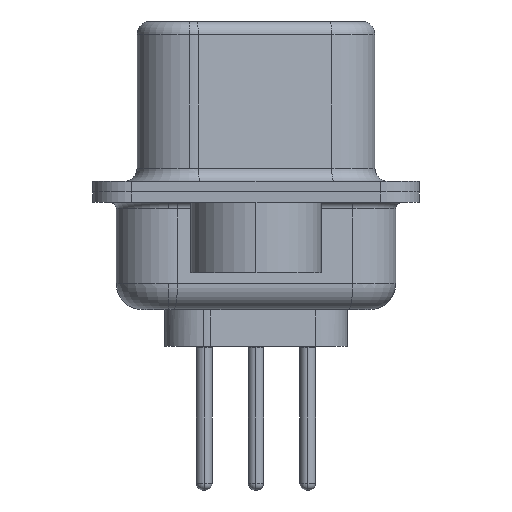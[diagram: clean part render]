
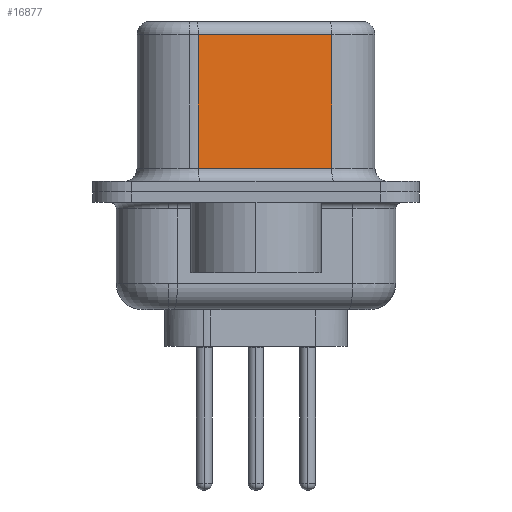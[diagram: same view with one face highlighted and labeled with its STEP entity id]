
A CAD part, left-side view. The second image highlights one B-rep face of the part: STEP entity #16877.
In plain terms, the highlighted planar face has unit normal (-0.985, -0.174, 0).
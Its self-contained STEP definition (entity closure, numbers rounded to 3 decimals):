
#751 = DIRECTION ( 'NONE',  ( 0.985, 0.174, 0. ) ) ;
#2518 = EDGE_CURVE ( 'NONE', #10097, #17260, #2590, .T. ) ;
#2590 = LINE ( 'NONE', #4401, #18952 ) ;
#2786 = ORIENTED_EDGE ( 'NONE', *, *, #15749, .F. ) ;
#3525 = CARTESIAN_POINT ( 'NONE',  ( 4.555, -2.897, 0.9 ) ) ;
#3633 = ORIENTED_EDGE ( 'NONE', *, *, #13662, .T. ) ;
#4401 = CARTESIAN_POINT ( 'NONE',  ( 4.555, -2.897, 0.9 ) ) ;
#5691 = CARTESIAN_POINT ( 'NONE',  ( 4.555, -2.897, 6.52 ) ) ;
#7303 = CARTESIAN_POINT ( 'NONE',  ( 4.555, -2.897, 6.02 ) ) ;
#7858 = ORIENTED_EDGE ( 'NONE', *, *, #2518, .T. ) ;
#8442 = VECTOR ( 'NONE', #16738, 1000. ) ;
#8526 = CARTESIAN_POINT ( 'NONE',  ( 3.655, 2.203, 6.02 ) ) ;
#8608 = DIRECTION ( 'NONE',  ( -0.174, 0.985, 0. ) ) ;
#9135 = EDGE_LOOP ( 'NONE', ( #2786, #3633, #17590, #7858 ) ) ;
#10097 = VERTEX_POINT ( 'NONE', #19469 ) ;
#12008 = CARTESIAN_POINT ( 'NONE',  ( 4.555, -2.897, 6.52 ) ) ;
#12025 = LINE ( 'NONE', #12008, #19852 ) ;
#12046 = DIRECTION ( 'NONE',  ( -0.174, 0.985, 0. ) ) ;
#12749 = VERTEX_POINT ( 'NONE', #7303 ) ;
#13154 = AXIS2_PLACEMENT_3D ( 'NONE', #5691, #751, #12046 ) ;
#13632 = CARTESIAN_POINT ( 'NONE',  ( 3.655, 2.203, 6.52 ) ) ;
#13662 = EDGE_CURVE ( 'NONE', #12749, #17934, #15908, .T. ) ;
#14040 = DIRECTION ( 'NONE',  ( 0.174, -0.985, 0. ) ) ;
#15227 = FACE_OUTER_BOUND ( 'NONE', #9135, .T. ) ;
#15749 = EDGE_CURVE ( 'NONE', #12749, #17260, #12025, .T. ) ;
#15908 = LINE ( 'NONE', #19600, #19550 ) ;
#16738 = DIRECTION ( 'NONE',  ( 0., 0., -1. ) ) ;
#16834 = LINE ( 'NONE', #13632, #8442 ) ;
#16877 = ADVANCED_FACE ( 'NONE', ( #15227 ), #18266, .F. ) ;
#17260 = VERTEX_POINT ( 'NONE', #3525 ) ;
#17590 = ORIENTED_EDGE ( 'NONE', *, *, #18074, .T. ) ;
#17934 = VERTEX_POINT ( 'NONE', #8526 ) ;
#18074 = EDGE_CURVE ( 'NONE', #17934, #10097, #16834, .T. ) ;
#18266 = PLANE ( 'NONE',  #13154 ) ;
#18952 = VECTOR ( 'NONE', #14040, 1000. ) ;
#19469 = CARTESIAN_POINT ( 'NONE',  ( 3.655, 2.203, 0.9 ) ) ;
#19550 = VECTOR ( 'NONE', #8608, 1000. ) ;
#19600 = CARTESIAN_POINT ( 'NONE',  ( 4.555, -2.897, 6.02 ) ) ;
#19852 = VECTOR ( 'NONE', #20131, 1000. ) ;
#20131 = DIRECTION ( 'NONE',  ( 0., 0., -1. ) ) ;
